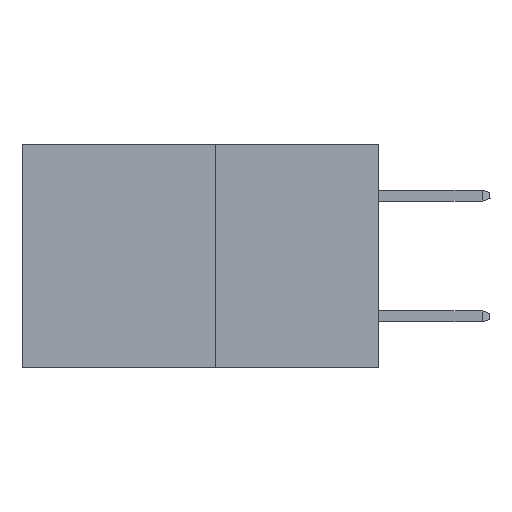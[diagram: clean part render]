
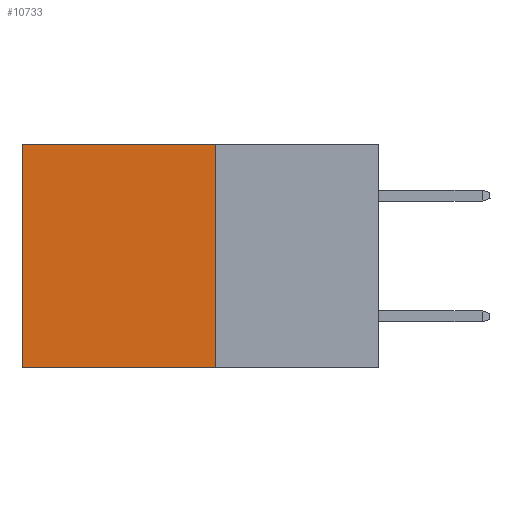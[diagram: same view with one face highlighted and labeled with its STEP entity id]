
A CAD part, left-side view. The second image highlights one B-rep face of the part: STEP entity #10733.
In plain terms, the highlighted planar face has unit normal (-1, 0, 0).
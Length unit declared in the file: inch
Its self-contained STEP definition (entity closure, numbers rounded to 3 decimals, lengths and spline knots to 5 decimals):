
#203 = ORIENTED_EDGE ( 'NONE', *, *, #13014, .F. ) ;
#436 = VECTOR ( 'NONE', #16740, 39.37008 ) ;
#446 = ORIENTED_EDGE ( 'NONE', *, *, #5302, .T. ) ;
#761 = VECTOR ( 'NONE', #9493, 39.37008 ) ;
#1177 = ORIENTED_EDGE ( 'NONE', *, *, #19164, .T. ) ;
#1245 = FACE_OUTER_BOUND ( 'NONE', #17450, .T. ) ;
#1729 = CARTESIAN_POINT ( 'NONE',  ( 0.277, 0.27, 0. ) ) ;
#4190 = DIRECTION ( 'NONE',  ( 0., 1., 0. ) ) ;
#4434 = LINE ( 'NONE', #9255, #8014 ) ;
#5302 = EDGE_CURVE ( 'NONE', #6200, #8156, #10731, .T. ) ;
#6200 = VERTEX_POINT ( 'NONE', #1729 ) ;
#6215 = VECTOR ( 'NONE', #4190, 39.37008 ) ;
#6350 = CARTESIAN_POINT ( 'NONE',  ( 0.277, 0.59, -0.37 ) ) ;
#7128 = DIRECTION ( 'NONE',  ( 1., 0., 0. ) ) ;
#7153 = CARTESIAN_POINT ( 'NONE',  ( 0.277, 0.27, -0.37 ) ) ;
#8014 = VECTOR ( 'NONE', #13796, 39.37008 ) ;
#8156 = VERTEX_POINT ( 'NONE', #14175 ) ;
#8664 = DIRECTION ( 'NONE',  ( 0., 0., -1. ) ) ;
#9096 = VERTEX_POINT ( 'NONE', #14002 ) ;
#9255 = CARTESIAN_POINT ( 'NONE',  ( 0.277, 0.27, -0.37 ) ) ;
#9493 = DIRECTION ( 'NONE',  ( 0., 0., -1. ) ) ;
#10083 = CARTESIAN_POINT ( 'NONE',  ( 0.277, 0.27, 0. ) ) ;
#10731 = LINE ( 'NONE', #10083, #6215 ) ;
#10733 = ADVANCED_FACE ( 'NONE', ( #1245 ), #18768, .F. ) ;
#11018 = CARTESIAN_POINT ( 'NONE',  ( 0.277, 0.27, -0.37 ) ) ;
#12034 = LINE ( 'NONE', #15772, #436 ) ;
#12260 = VERTEX_POINT ( 'NONE', #11018 ) ;
#13014 = EDGE_CURVE ( 'NONE', #12260, #9096, #12034, .T. ) ;
#13295 = LINE ( 'NONE', #6350, #761 ) ;
#13796 = DIRECTION ( 'NONE',  ( 0., 0., -1. ) ) ;
#14002 = CARTESIAN_POINT ( 'NONE',  ( 0.277, 0.59, -0.37 ) ) ;
#14003 = AXIS2_PLACEMENT_3D ( 'NONE', #7153, #7128, #8664 ) ;
#14175 = CARTESIAN_POINT ( 'NONE',  ( 0.277, 0.59, 0. ) ) ;
#15772 = CARTESIAN_POINT ( 'NONE',  ( 0.277, 0.27, -0.37 ) ) ;
#16740 = DIRECTION ( 'NONE',  ( 0., 1., 0. ) ) ;
#16963 = EDGE_CURVE ( 'NONE', #6200, #12260, #4434, .T. ) ;
#17450 = EDGE_LOOP ( 'NONE', ( #1177, #203, #18339, #446 ) ) ;
#18339 = ORIENTED_EDGE ( 'NONE', *, *, #16963, .F. ) ;
#18768 = PLANE ( 'NONE',  #14003 ) ;
#19164 = EDGE_CURVE ( 'NONE', #8156, #9096, #13295, .T. ) ;
